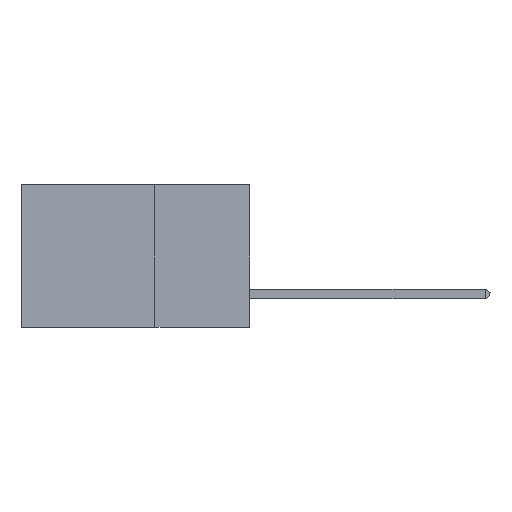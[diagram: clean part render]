
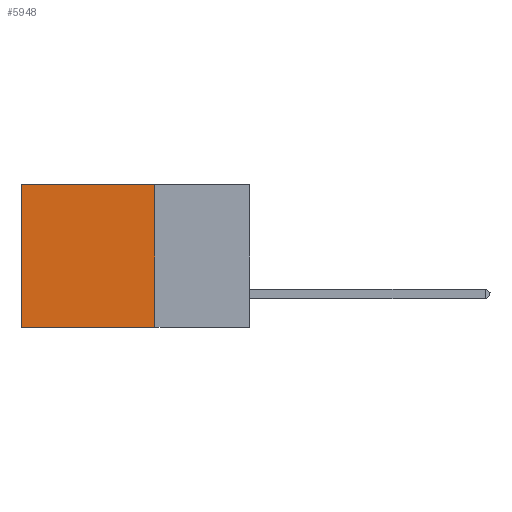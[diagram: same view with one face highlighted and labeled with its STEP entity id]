
A CAD part, left-side view. The second image highlights one B-rep face of the part: STEP entity #5948.
In plain terms, the highlighted planar face has unit normal (-1, 0, 0).
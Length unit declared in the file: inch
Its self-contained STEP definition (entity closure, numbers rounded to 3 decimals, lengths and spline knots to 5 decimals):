
#436 = VECTOR ( 'NONE', #11200, 39.37008 ) ;
#446 = CARTESIAN_POINT ( 'NONE',  ( 0.2875, 0.6, -0.375 ) ) ;
#844 = CARTESIAN_POINT ( 'NONE',  ( 0.2875, 0.25, -0.375 ) ) ;
#1971 = EDGE_CURVE ( 'NONE', #8676, #14395, #2725, .T. ) ;
#2725 = LINE ( 'NONE', #9455, #14981 ) ;
#3071 = DIRECTION ( 'NONE',  ( 0., 1., 0. ) ) ;
#3584 = EDGE_LOOP ( 'NONE', ( #5759, #8686, #11262, #14422 ) ) ;
#3908 = CARTESIAN_POINT ( 'NONE',  ( 0.2875, 0.25, -0.375 ) ) ;
#5691 = EDGE_CURVE ( 'NONE', #6377, #11985, #8844, .T. ) ;
#5759 = ORIENTED_EDGE ( 'NONE', *, *, #8160, .T. ) ;
#5948 = ADVANCED_FACE ( 'NONE', ( #8133 ), #12706, .F. ) ;
#6377 = VERTEX_POINT ( 'NONE', #844 ) ;
#6605 = CARTESIAN_POINT ( 'NONE',  ( 0.2875, 0.25, 0. ) ) ;
#7161 = DIRECTION ( 'NONE',  ( 0., 0., -1. ) ) ;
#7222 = CARTESIAN_POINT ( 'NONE',  ( 0.2875, 0.25, -0.375 ) ) ;
#7740 = CARTESIAN_POINT ( 'NONE',  ( 0.2875, 0.25, -0.375 ) ) ;
#8133 = FACE_OUTER_BOUND ( 'NONE', #3584, .T. ) ;
#8160 = EDGE_CURVE ( 'NONE', #14395, #11985, #12236, .T. ) ;
#8676 = VERTEX_POINT ( 'NONE', #6605 ) ;
#8686 = ORIENTED_EDGE ( 'NONE', *, *, #5691, .F. ) ;
#8844 = LINE ( 'NONE', #7740, #9059 ) ;
#9059 = VECTOR ( 'NONE', #3071, 39.37008 ) ;
#9455 = CARTESIAN_POINT ( 'NONE',  ( 0.2875, 0.25, 0. ) ) ;
#10576 = CARTESIAN_POINT ( 'NONE',  ( 0.2875, 0.6, 0. ) ) ;
#11200 = DIRECTION ( 'NONE',  ( 0., 0., -1. ) ) ;
#11262 = ORIENTED_EDGE ( 'NONE', *, *, #18099, .F. ) ;
#11985 = VERTEX_POINT ( 'NONE', #446 ) ;
#12236 = LINE ( 'NONE', #12614, #436 ) ;
#12614 = CARTESIAN_POINT ( 'NONE',  ( 0.2875, 0.6, -0.375 ) ) ;
#12706 = PLANE ( 'NONE',  #19063 ) ;
#13855 = DIRECTION ( 'NONE',  ( 0., 1., 0. ) ) ;
#14212 = DIRECTION ( 'NONE',  ( 0., 0., -1. ) ) ;
#14395 = VERTEX_POINT ( 'NONE', #10576 ) ;
#14422 = ORIENTED_EDGE ( 'NONE', *, *, #1971, .T. ) ;
#14981 = VECTOR ( 'NONE', #13855, 39.37008 ) ;
#15812 = VECTOR ( 'NONE', #7161, 39.37008 ) ;
#17095 = DIRECTION ( 'NONE',  ( 1., 0., 0. ) ) ;
#18099 = EDGE_CURVE ( 'NONE', #8676, #6377, #18365, .T. ) ;
#18365 = LINE ( 'NONE', #7222, #15812 ) ;
#19063 = AXIS2_PLACEMENT_3D ( 'NONE', #3908, #17095, #14212 ) ;
